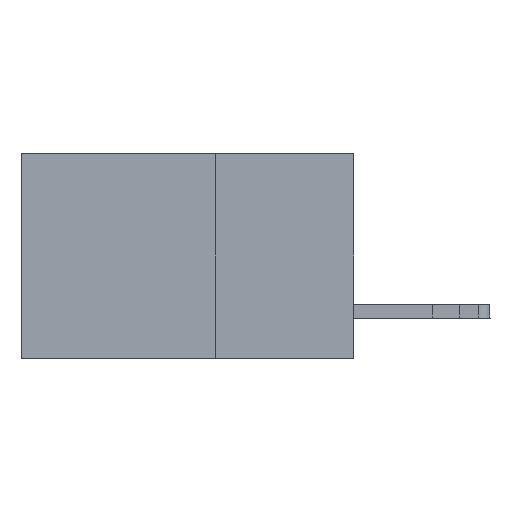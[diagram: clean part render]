
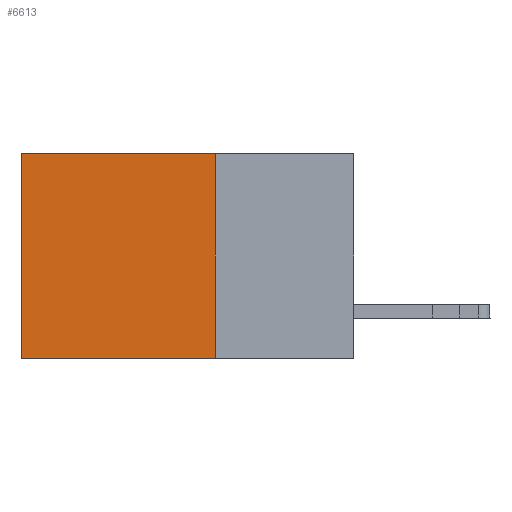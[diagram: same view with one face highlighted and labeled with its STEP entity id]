
A CAD part, left-side view. The second image highlights one B-rep face of the part: STEP entity #6613.
In plain terms, the highlighted planar face has unit normal (-1, 0, 0).
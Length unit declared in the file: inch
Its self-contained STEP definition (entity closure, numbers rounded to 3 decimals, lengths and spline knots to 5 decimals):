
#612 = DIRECTION ( 'NONE',  ( 0., 0., -1. ) ) ;
#757 = DIRECTION ( 'NONE',  ( 0., 1., 0. ) ) ;
#2333 = VERTEX_POINT ( 'NONE', #26191 ) ;
#2662 = VERTEX_POINT ( 'NONE', #15307 ) ;
#5118 = ORIENTED_EDGE ( 'NONE', *, *, #31537, .T. ) ;
#5678 = PLANE ( 'NONE',  #22671 ) ;
#5723 = VECTOR ( 'NONE', #17701, 39.37008 ) ;
#5897 = ORIENTED_EDGE ( 'NONE', *, *, #10404, .F. ) ;
#6482 = LINE ( 'NONE', #23624, #12479 ) ;
#6613 = ADVANCED_FACE ( 'NONE', ( #13383 ), #5678, .F. ) ;
#6783 = LINE ( 'NONE', #17100, #32767 ) ;
#9058 = VECTOR ( 'NONE', #612, 39.37008 ) ;
#9453 = DIRECTION ( 'NONE',  ( 0., 1., 0. ) ) ;
#10404 = EDGE_CURVE ( 'NONE', #21688, #12140, #19352, .T. ) ;
#10808 = DIRECTION ( 'NONE',  ( 0., 0., -1. ) ) ;
#10817 = CARTESIAN_POINT ( 'NONE',  ( 0.2875, 0.6, 0. ) ) ;
#10876 = ORIENTED_EDGE ( 'NONE', *, *, #16184, .F. ) ;
#12140 = VERTEX_POINT ( 'NONE', #14363 ) ;
#12479 = VECTOR ( 'NONE', #757, 39.37008 ) ;
#13287 = CARTESIAN_POINT ( 'NONE',  ( 0.2875, 0.25, 0. ) ) ;
#13383 = FACE_OUTER_BOUND ( 'NONE', #31749, .T. ) ;
#14363 = CARTESIAN_POINT ( 'NONE',  ( 0.2875, 0.25, -0.37 ) ) ;
#15129 = CARTESIAN_POINT ( 'NONE',  ( 0.2875, 0.25, 0. ) ) ;
#15307 = CARTESIAN_POINT ( 'NONE',  ( 0.2875, 0.6, -0.37 ) ) ;
#16184 = EDGE_CURVE ( 'NONE', #12140, #2662, #6482, .T. ) ;
#17100 = CARTESIAN_POINT ( 'NONE',  ( 0.2875, 0.25, 0. ) ) ;
#17701 = DIRECTION ( 'NONE',  ( 0., 0., -1. ) ) ;
#18945 = CARTESIAN_POINT ( 'NONE',  ( 0.2875, 0.25, 0. ) ) ;
#19352 = LINE ( 'NONE', #15129, #5723 ) ;
#21688 = VERTEX_POINT ( 'NONE', #18945 ) ;
#22588 = LINE ( 'NONE', #10817, #9058 ) ;
#22671 = AXIS2_PLACEMENT_3D ( 'NONE', #13287, #25981, #10808 ) ;
#23272 = ORIENTED_EDGE ( 'NONE', *, *, #25045, .T. ) ;
#23624 = CARTESIAN_POINT ( 'NONE',  ( 0.2875, 0.25, -0.37 ) ) ;
#25045 = EDGE_CURVE ( 'NONE', #21688, #2333, #6783, .T. ) ;
#25981 = DIRECTION ( 'NONE',  ( 1., 0., 0. ) ) ;
#26191 = CARTESIAN_POINT ( 'NONE',  ( 0.2875, 0.6, 0. ) ) ;
#31537 = EDGE_CURVE ( 'NONE', #2333, #2662, #22588, .T. ) ;
#31749 = EDGE_LOOP ( 'NONE', ( #5118, #10876, #5897, #23272 ) ) ;
#32767 = VECTOR ( 'NONE', #9453, 39.37008 ) ;
